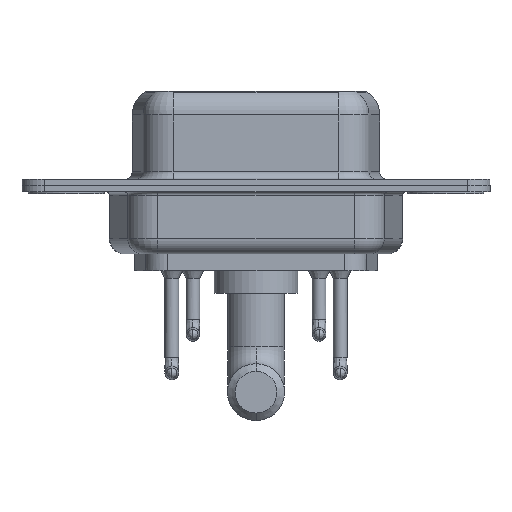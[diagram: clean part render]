
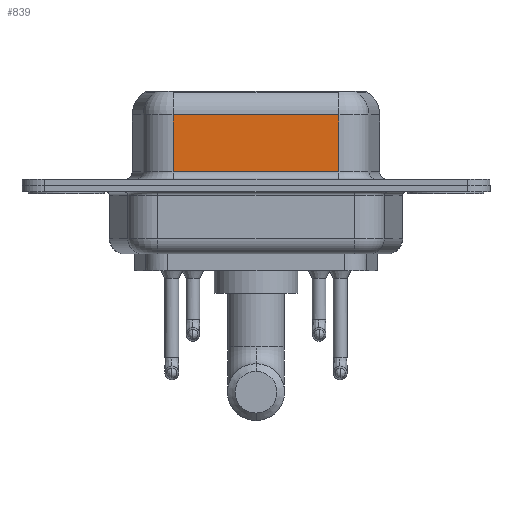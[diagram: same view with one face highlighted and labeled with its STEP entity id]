
A CAD part, front view. The second image highlights one B-rep face of the part: STEP entity #839.
In plain terms, the highlighted planar face has unit normal (0, -1, 0).
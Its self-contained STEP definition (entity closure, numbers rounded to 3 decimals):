
#839 = ADVANCED_FACE ( 'NONE', ( #13296 ), #7716, .F. ) ;
#1003 = DIRECTION ( 'NONE',  ( 0., 0., -1. ) ) ;
#1322 = EDGE_LOOP ( 'NONE', ( #7586, #2358, #8593, #6274 ) ) ;
#1472 = AXIS2_PLACEMENT_3D ( 'NONE', #12195, #11168, #5577 ) ;
#2358 = ORIENTED_EDGE ( 'NONE', *, *, #11019, .T. ) ;
#3469 = VERTEX_POINT ( 'NONE', #10363 ) ;
#3539 = VERTEX_POINT ( 'NONE', #8311 ) ;
#3748 = CARTESIAN_POINT ( 'NONE',  ( 17.962, -3.95, 0.9 ) ) ;
#4470 = CARTESIAN_POINT ( 'NONE',  ( 17.962, -3.95, 4.65 ) ) ;
#4562 = VERTEX_POINT ( 'NONE', #13743 ) ;
#5002 = DIRECTION ( 'NONE',  ( 0., 0., -1. ) ) ;
#5577 = DIRECTION ( 'NONE',  ( -1., 0., 0. ) ) ;
#5708 = DIRECTION ( 'NONE',  ( -1., 0., 0. ) ) ;
#6274 = ORIENTED_EDGE ( 'NONE', *, *, #9599, .T. ) ;
#6582 = LINE ( 'NONE', #10169, #11873 ) ;
#6733 = VECTOR ( 'NONE', #5708, 1000. ) ;
#6883 = LINE ( 'NONE', #4470, #6733 ) ;
#7586 = ORIENTED_EDGE ( 'NONE', *, *, #11465, .F. ) ;
#7716 = PLANE ( 'NONE',  #1472 ) ;
#8224 = DIRECTION ( 'NONE',  ( 1., 0., 0. ) ) ;
#8311 = CARTESIAN_POINT ( 'NONE',  ( 7.038, -3.95, 0.9 ) ) ;
#8459 = CARTESIAN_POINT ( 'NONE',  ( 7.038, -3.95, 6.4 ) ) ;
#8593 = ORIENTED_EDGE ( 'NONE', *, *, #10899, .T. ) ;
#9599 = EDGE_CURVE ( 'NONE', #3539, #4562, #13810, .T. ) ;
#9769 = VECTOR ( 'NONE', #5002, 1000. ) ;
#10169 = CARTESIAN_POINT ( 'NONE',  ( 17.962, -3.95, 6.4 ) ) ;
#10363 = CARTESIAN_POINT ( 'NONE',  ( 7.038, -3.95, 4.65 ) ) ;
#10476 = CARTESIAN_POINT ( 'NONE',  ( 17.962, -3.95, 4.65 ) ) ;
#10899 = EDGE_CURVE ( 'NONE', #3469, #3539, #12112, .T. ) ;
#10918 = VECTOR ( 'NONE', #8224, 1000. ) ;
#11019 = EDGE_CURVE ( 'NONE', #11178, #3469, #6883, .T. ) ;
#11168 = DIRECTION ( 'NONE',  ( 0., 1., 0. ) ) ;
#11178 = VERTEX_POINT ( 'NONE', #10476 ) ;
#11465 = EDGE_CURVE ( 'NONE', #11178, #4562, #6582, .T. ) ;
#11873 = VECTOR ( 'NONE', #1003, 1000. ) ;
#12112 = LINE ( 'NONE', #8459, #9769 ) ;
#12195 = CARTESIAN_POINT ( 'NONE',  ( 17.962, -3.95, 6.4 ) ) ;
#13296 = FACE_OUTER_BOUND ( 'NONE', #1322, .T. ) ;
#13743 = CARTESIAN_POINT ( 'NONE',  ( 17.962, -3.95, 0.9 ) ) ;
#13810 = LINE ( 'NONE', #3748, #10918 ) ;
